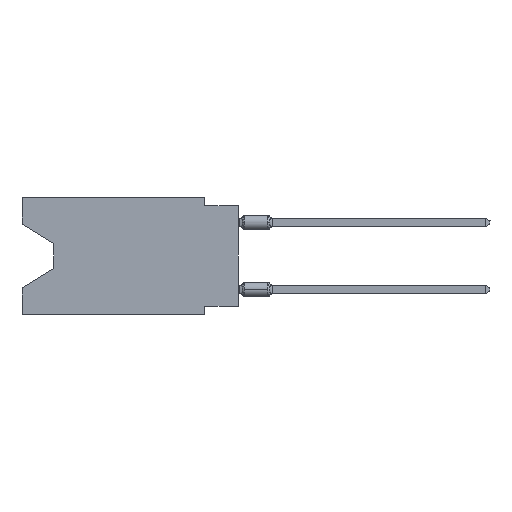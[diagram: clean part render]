
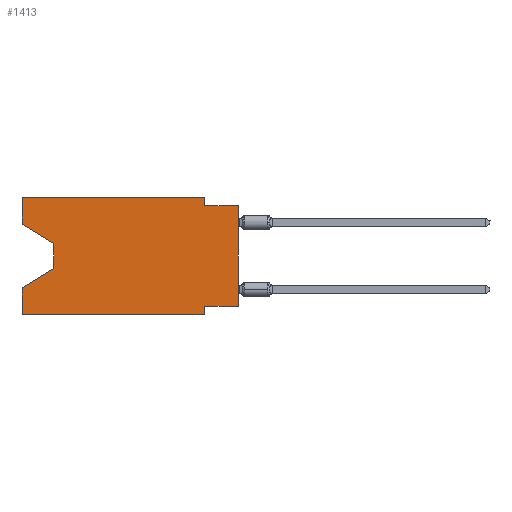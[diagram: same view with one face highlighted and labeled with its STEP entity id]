
A CAD part, left-side view. The second image highlights one B-rep face of the part: STEP entity #1413.
In plain terms, the highlighted planar face has unit normal (-1, 0, 0).
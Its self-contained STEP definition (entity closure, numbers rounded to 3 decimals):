
#67 = VERTEX_POINT ( 'NONE', #16000 ) ;
#728 = EDGE_CURVE ( 'NONE', #17218, #49402, #63999, .T. ) ;
#1413 = ADVANCED_FACE ( 'NONE', ( #19598 ), #36363, .F. ) ;
#2254 = VERTEX_POINT ( 'NONE', #27462 ) ;
#6134 = CARTESIAN_POINT ( 'NONE',  ( 0., 16.383, -2.038 ) ) ;
#6389 = CARTESIAN_POINT ( 'NONE',  ( 0., 2.54, 0. ) ) ;
#7128 = VERTEX_POINT ( 'NONE', #38799 ) ;
#7135 = CARTESIAN_POINT ( 'NONE',  ( 0., 16.383, -8.89 ) ) ;
#7802 = VECTOR ( 'NONE', #13227, 1000. ) ;
#7846 = LINE ( 'NONE', #8953, #56098 ) ;
#8555 = DIRECTION ( 'NONE',  ( 0., 0., 1. ) ) ;
#8638 = ORIENTED_EDGE ( 'NONE', *, *, #59051, .F. ) ;
#8739 = AXIS2_PLACEMENT_3D ( 'NONE', #59072, #35979, #58687 ) ;
#8953 = CARTESIAN_POINT ( 'NONE',  ( 0., 16.383, 0. ) ) ;
#10372 = VECTOR ( 'NONE', #16079, 1000. ) ;
#10694 = VECTOR ( 'NONE', #62493, 1000. ) ;
#10954 = VERTEX_POINT ( 'NONE', #63256 ) ;
#12564 = DIRECTION ( 'NONE',  ( 0., 1., 0. ) ) ;
#12617 = ORIENTED_EDGE ( 'NONE', *, *, #728, .F. ) ;
#13227 = DIRECTION ( 'NONE',  ( 0., -1., 0. ) ) ;
#13399 = VECTOR ( 'NONE', #69966, 1000. ) ;
#13459 = EDGE_CURVE ( 'NONE', #41802, #10954, #69485, .T. ) ;
#15838 = EDGE_CURVE ( 'NONE', #67, #23892, #32031, .T. ) ;
#15943 = CARTESIAN_POINT ( 'NONE',  ( 0., 16.383, 0. ) ) ;
#16000 = CARTESIAN_POINT ( 'NONE',  ( 0., 13.97, -5.385 ) ) ;
#16079 = DIRECTION ( 'NONE',  ( 0., 0., -1. ) ) ;
#16854 = VECTOR ( 'NONE', #51401, 1000. ) ;
#17218 = VERTEX_POINT ( 'NONE', #70308 ) ;
#17863 = LINE ( 'NONE', #33889, #16854 ) ;
#18208 = EDGE_CURVE ( 'NONE', #69099, #10954, #36889, .T. ) ;
#19263 = EDGE_CURVE ( 'NONE', #69099, #2254, #25521, .T. ) ;
#19598 = FACE_OUTER_BOUND ( 'NONE', #22033, .T. ) ;
#19945 = CARTESIAN_POINT ( 'NONE',  ( 0., 0., -8.255 ) ) ;
#20482 = CARTESIAN_POINT ( 'NONE',  ( 0., 0., 0. ) ) ;
#20509 = DIRECTION ( 'NONE',  ( 0., -1., 0. ) ) ;
#20694 = ORIENTED_EDGE ( 'NONE', *, *, #37936, .F. ) ;
#22033 = EDGE_LOOP ( 'NONE', ( #61822, #45058, #57038, #31799, #56996, #42882, #59260, #25123, #33721, #20694, #8638, #12617 ) ) ;
#23892 = VERTEX_POINT ( 'NONE', #47292 ) ;
#24972 = CARTESIAN_POINT ( 'NONE',  ( 0., 16.383, 0. ) ) ;
#25123 = ORIENTED_EDGE ( 'NONE', *, *, #18208, .T. ) ;
#25521 = LINE ( 'NONE', #19945, #72698 ) ;
#26063 = VECTOR ( 'NONE', #28871, 1000. ) ;
#26793 = CARTESIAN_POINT ( 'NONE',  ( 0., 13.97, -5.385 ) ) ;
#26813 = VERTEX_POINT ( 'NONE', #36385 ) ;
#27163 = DIRECTION ( 'NONE',  ( 0., 0.855, -0.519 ) ) ;
#27227 = VERTEX_POINT ( 'NONE', #7135 ) ;
#27462 = CARTESIAN_POINT ( 'NONE',  ( 0., 2.54, -8.255 ) ) ;
#28076 = LINE ( 'NONE', #66095, #42438 ) ;
#28096 = EDGE_CURVE ( 'NONE', #17218, #7128, #57190, .T. ) ;
#28871 = DIRECTION ( 'NONE',  ( 0., -0.855, -0.519 ) ) ;
#29675 = CARTESIAN_POINT ( 'NONE',  ( 0., 16.383, -8.89 ) ) ;
#30634 = EDGE_CURVE ( 'NONE', #27227, #26813, #42608, .T. ) ;
#31799 = ORIENTED_EDGE ( 'NONE', *, *, #37130, .F. ) ;
#32031 = LINE ( 'NONE', #26793, #69770 ) ;
#32482 = CARTESIAN_POINT ( 'NONE',  ( 0., 2.54, -8.89 ) ) ;
#32563 = DIRECTION ( 'NONE',  ( 0., 0., -1. ) ) ;
#33721 = ORIENTED_EDGE ( 'NONE', *, *, #13459, .F. ) ;
#33889 = CARTESIAN_POINT ( 'NONE',  ( 0., 13.97, -3.505 ) ) ;
#35979 = DIRECTION ( 'NONE',  ( 1., 0., 0. ) ) ;
#36363 = PLANE ( 'NONE',  #8739 ) ;
#36385 = CARTESIAN_POINT ( 'NONE',  ( 0., 2.54, -8.89 ) ) ;
#36889 = LINE ( 'NONE', #20482, #70088 ) ;
#37130 = EDGE_CURVE ( 'NONE', #27227, #23892, #44992, .T. ) ;
#37936 = EDGE_CURVE ( 'NONE', #60040, #41802, #28076, .T. ) ;
#38799 = CARTESIAN_POINT ( 'NONE',  ( 0., 13.97, -3.505 ) ) ;
#41802 = VERTEX_POINT ( 'NONE', #67031 ) ;
#41958 = CARTESIAN_POINT ( 'NONE',  ( 0., 0., -8.255 ) ) ;
#42438 = VECTOR ( 'NONE', #32563, 1000. ) ;
#42608 = LINE ( 'NONE', #29675, #51165 ) ;
#42882 = ORIENTED_EDGE ( 'NONE', *, *, #47515, .F. ) ;
#44023 = LINE ( 'NONE', #32482, #10372 ) ;
#44992 = LINE ( 'NONE', #15943, #10694 ) ;
#45058 = ORIENTED_EDGE ( 'NONE', *, *, #59207, .T. ) ;
#47292 = CARTESIAN_POINT ( 'NONE',  ( 0., 16.383, -6.852 ) ) ;
#47501 = CARTESIAN_POINT ( 'NONE',  ( 0., 0., -0.635 ) ) ;
#47515 = EDGE_CURVE ( 'NONE', #2254, #26813, #44023, .T. ) ;
#49402 = VERTEX_POINT ( 'NONE', #24972 ) ;
#51165 = VECTOR ( 'NONE', #69521, 1000. ) ;
#51401 = DIRECTION ( 'NONE',  ( 0., 0., -1. ) ) ;
#56098 = VECTOR ( 'NONE', #20509, 1000. ) ;
#56996 = ORIENTED_EDGE ( 'NONE', *, *, #30634, .T. ) ;
#57038 = ORIENTED_EDGE ( 'NONE', *, *, #15838, .T. ) ;
#57190 = LINE ( 'NONE', #6134, #26063 ) ;
#58687 = DIRECTION ( 'NONE',  ( 0., 0., -1. ) ) ;
#59051 = EDGE_CURVE ( 'NONE', #49402, #60040, #7846, .T. ) ;
#59072 = CARTESIAN_POINT ( 'NONE',  ( 0., 16.383, 0. ) ) ;
#59207 = EDGE_CURVE ( 'NONE', #7128, #67, #17863, .T. ) ;
#59260 = ORIENTED_EDGE ( 'NONE', *, *, #19263, .F. ) ;
#60040 = VERTEX_POINT ( 'NONE', #6389 ) ;
#61822 = ORIENTED_EDGE ( 'NONE', *, *, #28096, .T. ) ;
#62493 = DIRECTION ( 'NONE',  ( 0., 0., 1. ) ) ;
#62904 = CARTESIAN_POINT ( 'NONE',  ( 0., 16.383, 0. ) ) ;
#63256 = CARTESIAN_POINT ( 'NONE',  ( 0., 0., -0.635 ) ) ;
#63999 = LINE ( 'NONE', #62904, #13399 ) ;
#66095 = CARTESIAN_POINT ( 'NONE',  ( 0., 2.54, 0. ) ) ;
#67031 = CARTESIAN_POINT ( 'NONE',  ( 0., 2.54, -0.635 ) ) ;
#69099 = VERTEX_POINT ( 'NONE', #41958 ) ;
#69485 = LINE ( 'NONE', #47501, #7802 ) ;
#69521 = DIRECTION ( 'NONE',  ( 0., -1., 0. ) ) ;
#69770 = VECTOR ( 'NONE', #27163, 1000. ) ;
#69966 = DIRECTION ( 'NONE',  ( 0., 0., 1. ) ) ;
#70088 = VECTOR ( 'NONE', #8555, 1000. ) ;
#70308 = CARTESIAN_POINT ( 'NONE',  ( 0., 16.383, -2.038 ) ) ;
#72698 = VECTOR ( 'NONE', #12564, 1000. ) ;
